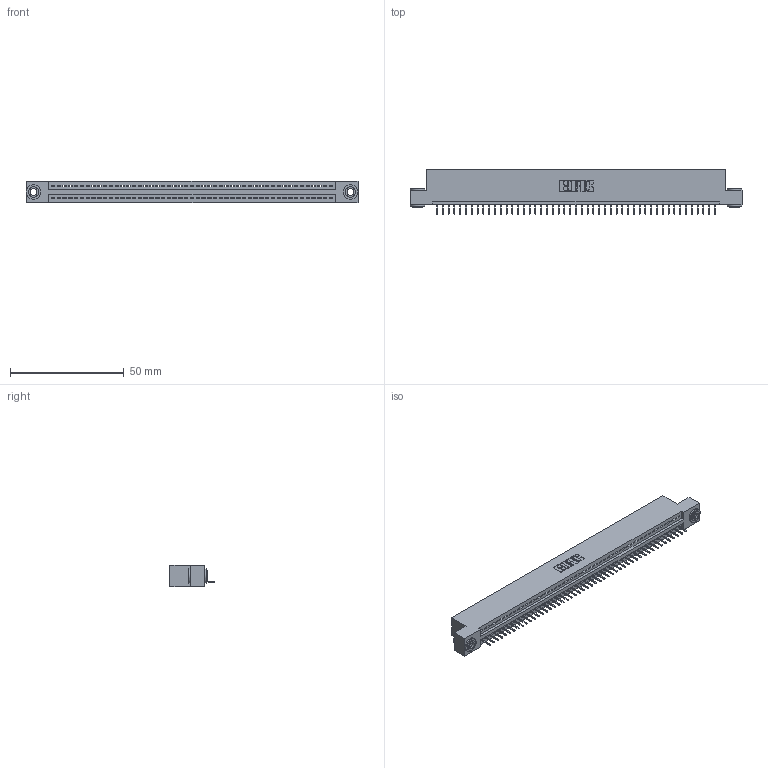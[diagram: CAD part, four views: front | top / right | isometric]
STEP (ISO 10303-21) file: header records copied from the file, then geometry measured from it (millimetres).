
FILE_DESCRIPTION (( 'STEP AP203' ), '1' );
FILE_NAME ('345-049-524-103.STEP', '2018-09-12T18:06:15', ( '' ), ( '' ), 'SwSTEP 2.0', 'SolidWorks 2016', '' );
FILE_SCHEMA (( 'CONFIG_CONTROL_DESIGN' ));
Length unit declared in the file: inch
Products named in the file (4): 345 Part_Flush Mounting Lugs - 0.156 Dia-TH; 345-292-001_345-293-124; 345-250-002_345-250-002-102; 345-049-524-103
Assembly tree (52 placements, depth 2):
  345-049-524-103
    345 Part_Flush Mounting Lugs - 0.156 Dia-TH
    345-292-001_345-293-124  x49
    345-250-002_345-250-002-102  x2
Bounding box: 145.67 x 19.35 x 9.4 mm (x, y, z)
Volume: 13719 mm3; surface area: 17922 mm2
Topology: 52 solids, 52 shells, 3202 faces, 9237 edges, 5958 vertices
Faces by surface type: plane 2344, cylinder 850, cone 8
Entity records: 36660 total; most frequent: CARTESIAN_POINT 6326, ORIENTED_EDGE 6302, DIRECTION 5547, EDGE_CURVE 3151, LINE 2803, VECTOR 2803, VERTEX_POINT 2094, AXIS2_PLACEMENT_3D 1372
